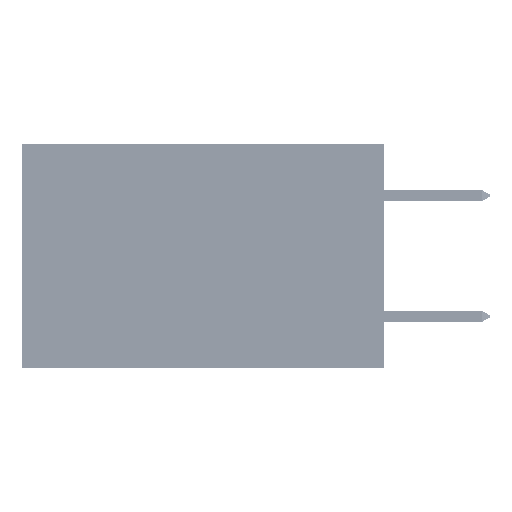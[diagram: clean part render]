
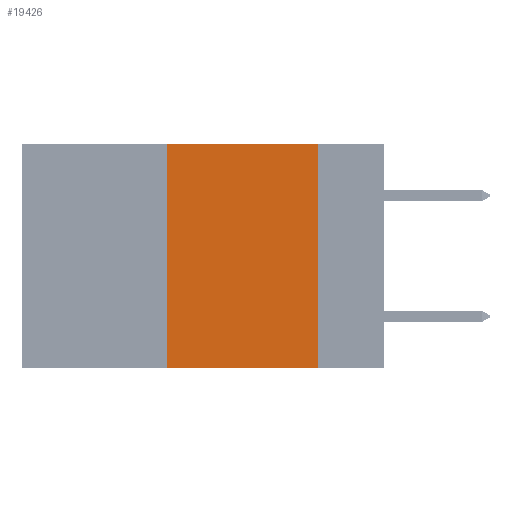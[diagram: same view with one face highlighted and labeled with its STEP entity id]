
A CAD part, left-side view. The second image highlights one B-rep face of the part: STEP entity #19426.
In plain terms, the highlighted planar face has unit normal (-1, 0, 0).
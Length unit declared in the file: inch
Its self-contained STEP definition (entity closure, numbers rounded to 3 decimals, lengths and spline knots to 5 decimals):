
#477 = EDGE_CURVE ( 'NONE', #31753, #30604, #28758, .T. ) ;
#1838 = CARTESIAN_POINT ( 'NONE',  ( 0., 0.11, 0. ) ) ;
#1854 = PLANE ( 'NONE',  #36897 ) ;
#2305 = LINE ( 'NONE', #25195, #11498 ) ;
#2618 = DIRECTION ( 'NONE',  ( 0., -1., 0. ) ) ;
#3090 = CARTESIAN_POINT ( 'NONE',  ( 0., 0.11, -0.37 ) ) ;
#3589 = VECTOR ( 'NONE', #2618, 39.37008 ) ;
#3661 = VECTOR ( 'NONE', #19506, 39.37008 ) ;
#5642 = DIRECTION ( 'NONE',  ( 0., 0., 1. ) ) ;
#8762 = DIRECTION ( 'NONE',  ( 0., -1., 0. ) ) ;
#9468 = EDGE_CURVE ( 'NONE', #31753, #27732, #2305, .T. ) ;
#10435 = EDGE_CURVE ( 'NONE', #28135, #30604, #33148, .T. ) ;
#10888 = CARTESIAN_POINT ( 'NONE',  ( 0., 0.36, -0.37 ) ) ;
#11498 = VECTOR ( 'NONE', #5642, 39.37008 ) ;
#14193 = DIRECTION ( 'NONE',  ( 0., 0., -1. ) ) ;
#14300 = ORIENTED_EDGE ( 'NONE', *, *, #477, .T. ) ;
#14646 = VECTOR ( 'NONE', #8762, 39.37008 ) ;
#19426 = ADVANCED_FACE ( 'NONE', ( #22593 ), #1854, .F. ) ;
#19506 = DIRECTION ( 'NONE',  ( 0., 0., -1. ) ) ;
#22593 = FACE_OUTER_BOUND ( 'NONE', #40660, .T. ) ;
#24701 = CARTESIAN_POINT ( 'NONE',  ( 0., 0.6, -0.37 ) ) ;
#24724 = ORIENTED_EDGE ( 'NONE', *, *, #9468, .F. ) ;
#25195 = CARTESIAN_POINT ( 'NONE',  ( 0., 0.36, 0. ) ) ;
#26130 = CARTESIAN_POINT ( 'NONE',  ( 0., 0.6, 0. ) ) ;
#26354 = CARTESIAN_POINT ( 'NONE',  ( 0., 0.6, 0. ) ) ;
#26732 = CARTESIAN_POINT ( 'NONE',  ( 0., 0.36, 0. ) ) ;
#27732 = VERTEX_POINT ( 'NONE', #26732 ) ;
#28135 = VERTEX_POINT ( 'NONE', #1838 ) ;
#28758 = LINE ( 'NONE', #24701, #14646 ) ;
#29969 = DIRECTION ( 'NONE',  ( 1., 0., 0. ) ) ;
#30604 = VERTEX_POINT ( 'NONE', #3090 ) ;
#31753 = VERTEX_POINT ( 'NONE', #10888 ) ;
#31838 = LINE ( 'NONE', #26130, #3589 ) ;
#33148 = LINE ( 'NONE', #42973, #3661 ) ;
#34776 = ORIENTED_EDGE ( 'NONE', *, *, #10435, .F. ) ;
#36897 = AXIS2_PLACEMENT_3D ( 'NONE', #26354, #29969, #14193 ) ;
#39373 = EDGE_CURVE ( 'NONE', #27732, #28135, #31838, .T. ) ;
#40660 = EDGE_LOOP ( 'NONE', ( #34776, #43395, #24724, #14300 ) ) ;
#42973 = CARTESIAN_POINT ( 'NONE',  ( 0., 0.11, 0. ) ) ;
#43395 = ORIENTED_EDGE ( 'NONE', *, *, #39373, .F. ) ;
